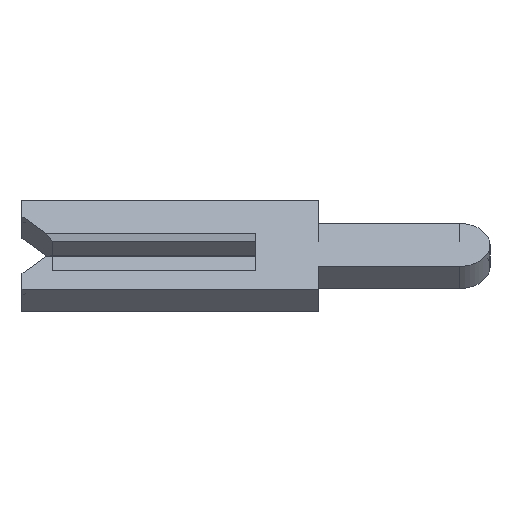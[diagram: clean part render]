
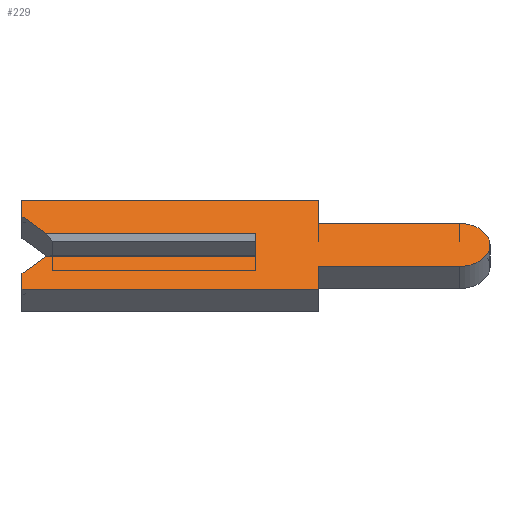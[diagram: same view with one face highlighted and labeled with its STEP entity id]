
A CAD part, left-side view. The second image highlights one B-rep face of the part: STEP entity #229.
In plain terms, the highlighted face is planar.
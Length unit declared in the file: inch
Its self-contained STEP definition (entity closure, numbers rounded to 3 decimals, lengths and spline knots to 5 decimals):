
#8 = VECTOR ( 'NONE', #1464, 39.37008 ) ;
#16 = VERTEX_POINT ( 'NONE', #170 ) ;
#38 = DIRECTION ( 'NONE',  ( 0., 0., -1. ) ) ;
#57 = LINE ( 'NONE', #1161, #306 ) ;
#60 = CARTESIAN_POINT ( 'NONE',  ( -0.01, 0.1305, 0.0065 ) ) ;
#98 = DIRECTION ( 'NONE',  ( 0., -1., 0. ) ) ;
#107 = AXIS2_PLACEMENT_3D ( 'NONE', #1669, #303, #141 ) ;
#113 = CARTESIAN_POINT ( 'NONE',  ( -0.01, -0.04, -0.0195 ) ) ;
#141 = DIRECTION ( 'NONE',  ( 0., 0., -1. ) ) ;
#158 = VERTEX_POINT ( 'NONE', #439 ) ;
#170 = CARTESIAN_POINT ( 'NONE',  ( -0.01, 0.15, 0.026 ) ) ;
#183 = EDGE_CURVE ( 'NONE', #193, #1508, #1684, .T. ) ;
#184 = DIRECTION ( 'NONE',  ( 0., 1., 0. ) ) ;
#193 = VERTEX_POINT ( 'NONE', #300 ) ;
#200 = ORIENTED_EDGE ( 'NONE', *, *, #1365, .F. ) ;
#223 = VECTOR ( 'NONE', #38, 39.37008 ) ;
#229 = ADVANCED_FACE ( 'NONE', ( #1646 ), #593, .F. ) ;
#241 = CARTESIAN_POINT ( 'NONE',  ( -0.01, 0.134, 0.01 ) ) ;
#244 = ORIENTED_EDGE ( 'NONE', *, *, #183, .F. ) ;
#261 = DIRECTION ( 'NONE',  ( 0., -1., 0. ) ) ;
#271 = VECTOR ( 'NONE', #1404, 39.37008 ) ;
#272 = CARTESIAN_POINT ( 'NONE',  ( -0.01, 0.15, -0.026 ) ) ;
#283 = LINE ( 'NONE', #1045, #1352 ) ;
#290 = VECTOR ( 'NONE', #261, 39.37008 ) ;
#300 = CARTESIAN_POINT ( 'NONE',  ( -0.01, 0.134, -0.01 ) ) ;
#303 = DIRECTION ( 'NONE',  ( 1., 0., 0. ) ) ;
#306 = VECTOR ( 'NONE', #1714, 39.37008 ) ;
#318 = CARTESIAN_POINT ( 'NONE',  ( -0.01, -0.04, 0.04 ) ) ;
#342 = CARTESIAN_POINT ( 'NONE',  ( -0.01, -0.04, -0.0195 ) ) ;
#374 = CARTESIAN_POINT ( 'NONE',  ( -0.01, 0.15, -0.026 ) ) ;
#386 = EDGE_CURVE ( 'NONE', #1043, #193, #57, .T. ) ;
#424 = VERTEX_POINT ( 'NONE', #740 ) ;
#430 = ORIENTED_EDGE ( 'NONE', *, *, #1021, .F. ) ;
#439 = CARTESIAN_POINT ( 'NONE',  ( -0.01, 0., 0.01 ) ) ;
#459 = VERTEX_POINT ( 'NONE', #342 ) ;
#464 = CARTESIAN_POINT ( 'NONE',  ( -0.01, 0.15, 0.01 ) ) ;
#470 = DIRECTION ( 'NONE',  ( 0., 0., -1. ) ) ;
#484 = EDGE_CURVE ( 'NONE', #1354, #1317, #1120, .T. ) ;
#497 = LINE ( 'NONE', #318, #271 ) ;
#560 = DIRECTION ( 'NONE',  ( 0., 0., 1. ) ) ;
#583 = ORIENTED_EDGE ( 'NONE', *, *, #745, .F. ) ;
#591 = DIRECTION ( 'NONE',  ( 0., -1., 0. ) ) ;
#593 = PLANE ( 'NONE',  #1550 ) ;
#599 = LINE ( 'NONE', #818, #965 ) ;
#604 = LINE ( 'NONE', #1078, #290 ) ;
#620 = EDGE_CURVE ( 'NONE', #1176, #158, #845, .T. ) ;
#660 = CARTESIAN_POINT ( 'NONE',  ( -0.01, -0.04, 0.0195 ) ) ;
#699 = VECTOR ( 'NONE', #184, 39.37008 ) ;
#706 = CARTESIAN_POINT ( 'NONE',  ( -0.01, -0.1305, -0.0195 ) ) ;
#710 = DIRECTION ( 'NONE',  ( 0., 0., 1. ) ) ;
#735 = ORIENTED_EDGE ( 'NONE', *, *, #484, .F. ) ;
#740 = CARTESIAN_POINT ( 'NONE',  ( -0.01, -0.1305, 0.0195 ) ) ;
#745 = EDGE_CURVE ( 'NONE', #1176, #16, #1003, .T. ) ;
#766 = DIRECTION ( 'NONE',  ( 0., 0., 1. ) ) ;
#783 = EDGE_CURVE ( 'NONE', #1317, #1043, #815, .T. ) ;
#787 = ORIENTED_EDGE ( 'NONE', *, *, #1635, .F. ) ;
#815 = LINE ( 'NONE', #374, #1203 ) ;
#818 = CARTESIAN_POINT ( 'NONE',  ( -0.01, 0.15, 0.026 ) ) ;
#839 = EDGE_CURVE ( 'NONE', #1069, #424, #283, .T. ) ;
#845 = LINE ( 'NONE', #464, #1048 ) ;
#847 = CARTESIAN_POINT ( 'NONE',  ( -0.01, 0., -0.01 ) ) ;
#852 = VERTEX_POINT ( 'NONE', #1743 ) ;
#859 = CARTESIAN_POINT ( 'NONE',  ( -0.01, -0.1305, 0. ) ) ;
#902 = ORIENTED_EDGE ( 'NONE', *, *, #839, .F. ) ;
#965 = VECTOR ( 'NONE', #560, 39.37008 ) ;
#989 = CARTESIAN_POINT ( 'NONE',  ( -0.01, -0.04, -0.04 ) ) ;
#1003 = LINE ( 'NONE', #60, #8 ) ;
#1021 = EDGE_CURVE ( 'NONE', #1340, #852, #604, .T. ) ;
#1042 = LINE ( 'NONE', #113, #1443 ) ;
#1043 = VERTEX_POINT ( 'NONE', #272 ) ;
#1045 = CARTESIAN_POINT ( 'NONE',  ( -0.01, -0.04, 0.0195 ) ) ;
#1047 = ORIENTED_EDGE ( 'NONE', *, *, #620, .T. ) ;
#1048 = VECTOR ( 'NONE', #1439, 39.37008 ) ;
#1069 = VERTEX_POINT ( 'NONE', #660 ) ;
#1076 = EDGE_LOOP ( 'NONE', ( #1047, #787, #244, #1665, #1452, #735, #1129, #1466, #1426, #902, #1227, #430, #200, #583 ) ) ;
#1078 = CARTESIAN_POINT ( 'NONE',  ( -0.01, 0.15, 0.04 ) ) ;
#1082 = EDGE_CURVE ( 'NONE', #1548, #459, #1042, .T. ) ;
#1088 = CARTESIAN_POINT ( 'NONE',  ( -0.01, 0.15, -0.04 ) ) ;
#1109 = CARTESIAN_POINT ( 'NONE',  ( -0.01, 0.15, 0.04 ) ) ;
#1120 = LINE ( 'NONE', #1149, #699 ) ;
#1129 = ORIENTED_EDGE ( 'NONE', *, *, #1495, .F. ) ;
#1149 = CARTESIAN_POINT ( 'NONE',  ( -0.01, 0.15, -0.04 ) ) ;
#1161 = CARTESIAN_POINT ( 'NONE',  ( -0.01, 0.1305, -0.0065 ) ) ;
#1176 = VERTEX_POINT ( 'NONE', #241 ) ;
#1203 = VECTOR ( 'NONE', #766, 39.37008 ) ;
#1209 = VECTOR ( 'NONE', #591, 39.37008 ) ;
#1227 = ORIENTED_EDGE ( 'NONE', *, *, #1704, .F. ) ;
#1250 = VECTOR ( 'NONE', #710, 39.37008 ) ;
#1283 = EDGE_CURVE ( 'NONE', #424, #1548, #1532, .T. ) ;
#1317 = VERTEX_POINT ( 'NONE', #1088 ) ;
#1340 = VERTEX_POINT ( 'NONE', #1109 ) ;
#1348 = DIRECTION ( 'NONE',  ( 0., 1., 0. ) ) ;
#1352 = VECTOR ( 'NONE', #98, 39.37008 ) ;
#1354 = VERTEX_POINT ( 'NONE', #1522 ) ;
#1365 = EDGE_CURVE ( 'NONE', #16, #1340, #599, .T. ) ;
#1404 = DIRECTION ( 'NONE',  ( 0., 0., -1. ) ) ;
#1421 = CARTESIAN_POINT ( 'NONE',  ( -0.01, -0.1305, -0.01 ) ) ;
#1426 = ORIENTED_EDGE ( 'NONE', *, *, #1283, .F. ) ;
#1439 = DIRECTION ( 'NONE',  ( 0., -1., 0. ) ) ;
#1443 = VECTOR ( 'NONE', #1348, 39.37008 ) ;
#1452 = ORIENTED_EDGE ( 'NONE', *, *, #783, .F. ) ;
#1464 = DIRECTION ( 'NONE',  ( 0., 0.707, 0.707 ) ) ;
#1466 = ORIENTED_EDGE ( 'NONE', *, *, #1082, .F. ) ;
#1495 = EDGE_CURVE ( 'NONE', #459, #1354, #1727, .T. ) ;
#1508 = VERTEX_POINT ( 'NONE', #847 ) ;
#1522 = CARTESIAN_POINT ( 'NONE',  ( -0.01, -0.04, -0.04 ) ) ;
#1532 = CIRCLE ( 'NONE', #107, 0.0195 ) ;
#1548 = VERTEX_POINT ( 'NONE', #706 ) ;
#1550 = AXIS2_PLACEMENT_3D ( 'NONE', #859, #1576, #470 ) ;
#1557 = CARTESIAN_POINT ( 'NONE',  ( -0.01, 0., 0.0065 ) ) ;
#1576 = DIRECTION ( 'NONE',  ( 1., 0., 0. ) ) ;
#1635 = EDGE_CURVE ( 'NONE', #1508, #158, #1702, .T. ) ;
#1646 = FACE_OUTER_BOUND ( 'NONE', #1076, .T. ) ;
#1665 = ORIENTED_EDGE ( 'NONE', *, *, #386, .F. ) ;
#1669 = CARTESIAN_POINT ( 'NONE',  ( -0.01, -0.1305, 0. ) ) ;
#1684 = LINE ( 'NONE', #1421, #1209 ) ;
#1702 = LINE ( 'NONE', #1557, #1250 ) ;
#1704 = EDGE_CURVE ( 'NONE', #852, #1069, #497, .T. ) ;
#1714 = DIRECTION ( 'NONE',  ( 0., -0.707, 0.707 ) ) ;
#1727 = LINE ( 'NONE', #989, #223 ) ;
#1743 = CARTESIAN_POINT ( 'NONE',  ( -0.01, -0.04, 0.04 ) ) ;
